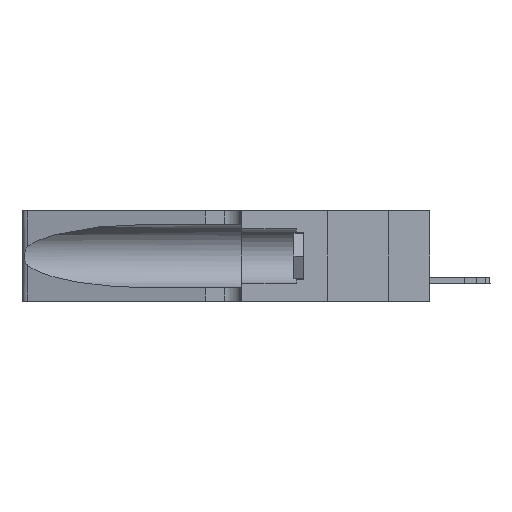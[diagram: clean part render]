
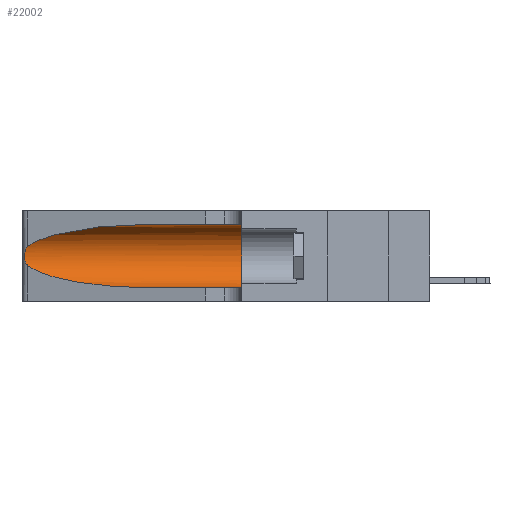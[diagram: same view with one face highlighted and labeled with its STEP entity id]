
A CAD part, left-side view. The second image highlights one B-rep face of the part: STEP entity #22002.
In plain terms, the highlighted cylindrical face has radius 3.308 mm (diameter 6.617 mm), a partial arc.
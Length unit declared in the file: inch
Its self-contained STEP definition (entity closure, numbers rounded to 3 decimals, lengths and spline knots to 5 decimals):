
#17 = VERTEX_POINT ( 'NONE', #12712 ) ;
#213 = DIRECTION ( 'NONE',  ( 0., -1., 0. ) ) ;
#479 = EDGE_CURVE ( 'NONE', #20281, #984, #17256, .T. ) ;
#749 = ORIENTED_EDGE ( 'NONE', *, *, #479, .T. ) ;
#856 = LINE ( 'NONE', #32258, #24901 ) ;
#984 = VERTEX_POINT ( 'NONE', #26047 ) ;
#2300 = CARTESIAN_POINT ( 'NONE',  ( 0.25487, 1.22718, 0.22369 ) ) ;
#3039 = VERTEX_POINT ( 'NONE', #5166 ) ;
#3386 = ORIENTED_EDGE ( 'NONE', *, *, #16225, .F. ) ;
#3826 = CYLINDRICAL_SURFACE ( 'NONE', #31068, 0.13025 ) ;
#4273 = CARTESIAN_POINT ( 'NONE',  ( 0.25639, 1.23184, 0.21858 ) ) ;
#5162 = CARTESIAN_POINT ( 'NONE',  ( 0.25487, 1.22718, 0.22369 ) ) ;
#5166 = CARTESIAN_POINT ( 'NONE',  ( 0.1305, 0.72297, 0.31525 ) ) ;
#5401 = CARTESIAN_POINT ( 'NONE',  ( 0.1305, 0.35, 0.185 ) ) ;
#6499 =( BOUNDED_CURVE ( )  B_SPLINE_CURVE ( 3, ( #25086, #12536, #12334, #2300 ),
 .UNSPECIFIED., .F., .F. ) 
 B_SPLINE_CURVE_WITH_KNOTS ( ( 4, 4 ),
 ( 1.5708, 2.84003 ),
 .UNSPECIFIED. ) 
 CURVE ( )  GEOMETRIC_REPRESENTATION_ITEM ( )  RATIONAL_B_SPLINE_CURVE ( ( 1., 0.87, 0.87, 1. ) ) 
 REPRESENTATION_ITEM ( '' )  );
#6549 = LINE ( 'NONE', #11494, #29011 ) ;
#6824 = CARTESIAN_POINT ( 'NONE',  ( 0.25639, 1.23186, 0.15144 ) ) ;
#9160 = CARTESIAN_POINT ( 'NONE',  ( 0.25856, 1.23593, 0.16098 ) ) ;
#9488 = EDGE_CURVE ( 'NONE', #3039, #32261, #6499, .T. ) ;
#9602 = CARTESIAN_POINT ( 'NONE',  ( 0.25555, 1.22994, 0.2215 ) ) ;
#9768 = AXIS2_PLACEMENT_3D ( 'NONE', #5401, #17800, #22736 ) ;
#10258 = DIRECTION ( 'NONE',  ( 0., 0., -1. ) ) ;
#11322 = FACE_OUTER_BOUND ( 'NONE', #22694, .T. ) ;
#11421 = ORIENTED_EDGE ( 'NONE', *, *, #18997, .T. ) ;
#11494 = CARTESIAN_POINT ( 'NONE',  ( 0.1305, 1.61858, 0.05475 ) ) ;
#11892 = CARTESIAN_POINT ( 'NONE',  ( 0.26075, 1.23896, 0.19203 ) ) ;
#12334 = CARTESIAN_POINT ( 'NONE',  ( 0.2373, 1.15595, 0.28018 ) ) ;
#12469 = ORIENTED_EDGE ( 'NONE', *, *, #9488, .T. ) ;
#12536 = CARTESIAN_POINT ( 'NONE',  ( 0.18966, 0.96281, 0.31525 ) ) ;
#12712 = CARTESIAN_POINT ( 'NONE',  ( 0.1305, 0.35, 0.05475 ) ) ;
#13003 = CARTESIAN_POINT ( 'NONE',  ( 0.1305, 1.61858, 0.185 ) ) ;
#13974 = CARTESIAN_POINT ( 'NONE',  ( 0.18966, 0.96281, 0.05475 ) ) ;
#14525 = CARTESIAN_POINT ( 'NONE',  ( 0.25487, 1.22718, 0.14631 ) ) ;
#16225 = EDGE_CURVE ( 'NONE', #3039, #25318, #856, .T. ) ;
#17011 = CARTESIAN_POINT ( 'NONE',  ( 0.25787, 1.23484, 0.2124 ) ) ;
#17225 = CARTESIAN_POINT ( 'NONE',  ( 0.26018, 1.23835, 0.19895 ) ) ;
#17256 =( BOUNDED_CURVE ( )  B_SPLINE_CURVE ( 3, ( #26917, #19258, #13974, #31950 ),
 .UNSPECIFIED., .F., .T. ) 
 B_SPLINE_CURVE_WITH_KNOTS ( ( 4, 4 ),
 ( 3.44316, 4.71239 ),
 .UNSPECIFIED. ) 
 CURVE ( )  GEOMETRIC_REPRESENTATION_ITEM ( )  RATIONAL_B_SPLINE_CURVE ( ( 1., 0.87, 0.87, 1. ) ) 
 REPRESENTATION_ITEM ( '' )  );
#17800 = DIRECTION ( 'NONE',  ( 0., 1., 0. ) ) ;
#18707 = EDGE_CURVE ( 'NONE', #25318, #17, #29409, .T. ) ;
#18997 = EDGE_CURVE ( 'NONE', #984, #17, #6549, .T. ) ;
#19258 = CARTESIAN_POINT ( 'NONE',  ( 0.2373, 1.15595, 0.08982 ) ) ;
#19422 = CARTESIAN_POINT ( 'NONE',  ( 0.25789, 1.23486, 0.15765 ) ) ;
#19640 = EDGE_CURVE ( 'NONE', #32261, #20281, #30836, .T. ) ;
#19795 = ORIENTED_EDGE ( 'NONE', *, *, #19640, .T. ) ;
#20281 = VERTEX_POINT ( 'NONE', #14525 ) ;
#21735 = CARTESIAN_POINT ( 'NONE',  ( 0.26017, 1.23833, 0.17102 ) ) ;
#21837 = CARTESIAN_POINT ( 'NONE',  ( 0.25555, 1.22993, 0.14849 ) ) ;
#21950 = CARTESIAN_POINT ( 'NONE',  ( 0.26075, 1.23896, 0.178 ) ) ;
#22002 = ADVANCED_FACE ( 'NONE', ( #11322 ), #3826, .F. ) ;
#22114 = DIRECTION ( 'NONE',  ( 0., -1., 0. ) ) ;
#22278 = CARTESIAN_POINT ( 'NONE',  ( 0.1305, 0.35, 0.31525 ) ) ;
#22694 = EDGE_LOOP ( 'NONE', ( #12469, #19795, #749, #11421, #23134, #3386 ) ) ;
#22736 = DIRECTION ( 'NONE',  ( 0., 0., 1. ) ) ;
#23134 = ORIENTED_EDGE ( 'NONE', *, *, #18707, .F. ) ;
#24235 = CARTESIAN_POINT ( 'NONE',  ( 0.25854, 1.2359, 0.20912 ) ) ;
#24657 = CARTESIAN_POINT ( 'NONE',  ( 0.25487, 1.22718, 0.22369 ) ) ;
#24901 = VECTOR ( 'NONE', #22114, 39.37008 ) ;
#25086 = CARTESIAN_POINT ( 'NONE',  ( 0.1305, 0.72297, 0.31525 ) ) ;
#25318 = VERTEX_POINT ( 'NONE', #22278 ) ;
#26047 = CARTESIAN_POINT ( 'NONE',  ( 0.1305, 0.72297, 0.05475 ) ) ;
#26917 = CARTESIAN_POINT ( 'NONE',  ( 0.25487, 1.22718, 0.14631 ) ) ;
#28772 = DIRECTION ( 'NONE',  ( 0., -1., 0. ) ) ;
#29011 = VECTOR ( 'NONE', #28772, 39.37008 ) ;
#29409 = CIRCLE ( 'NONE', #9768, 0.13025 ) ;
#29599 = CARTESIAN_POINT ( 'NONE',  ( 0.25487, 1.22718, 0.14631 ) ) ;
#30836 = B_SPLINE_CURVE_WITH_KNOTS ( 'NONE', 3,
 ( #24657, #9602, #4273, #17011, #24235, #17225, #11892, #21950, #21735, #9160, #19422, #6824, #21837, #29599 ),
 .UNSPECIFIED., .F., .F.,
 ( 4, 2, 2, 2, 2, 2, 4 ),
 ( 0., 0.00027, 0.00053, 0.00107, 0.0016, 0.00187, 0.00214 ),
 .UNSPECIFIED. ) ;
#31068 = AXIS2_PLACEMENT_3D ( 'NONE', #13003, #213, #10258 ) ;
#31950 = CARTESIAN_POINT ( 'NONE',  ( 0.1305, 0.72297, 0.05475 ) ) ;
#32258 = CARTESIAN_POINT ( 'NONE',  ( 0.1305, 1.61858, 0.31525 ) ) ;
#32261 = VERTEX_POINT ( 'NONE', #5162 ) ;
